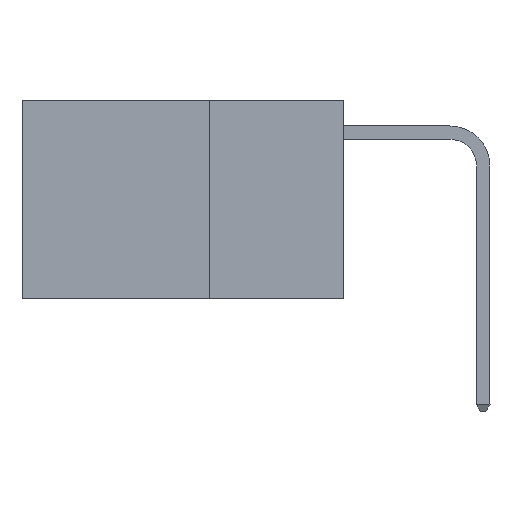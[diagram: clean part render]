
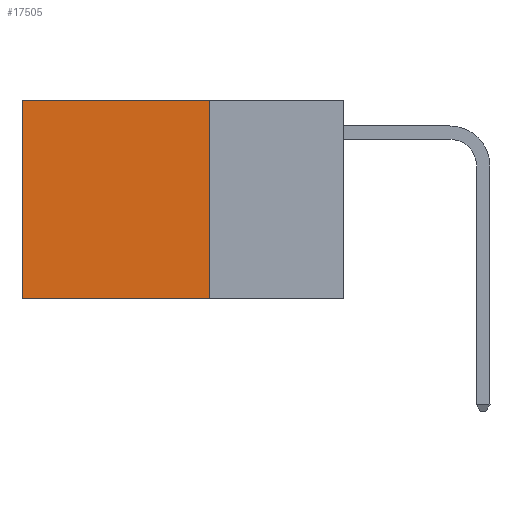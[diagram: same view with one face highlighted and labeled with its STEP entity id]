
A CAD part, left-side view. The second image highlights one B-rep face of the part: STEP entity #17505.
In plain terms, the highlighted planar face has unit normal (-1, 0, 0).
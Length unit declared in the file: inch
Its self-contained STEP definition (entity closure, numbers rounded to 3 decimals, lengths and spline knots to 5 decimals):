
#750 = ORIENTED_EDGE ( 'NONE', *, *, #7232, .T. ) ;
#976 = DIRECTION ( 'NONE',  ( 0., 1., 0. ) ) ;
#1484 = CARTESIAN_POINT ( 'NONE',  ( 0.2625, 0.25, 0. ) ) ;
#1677 = EDGE_LOOP ( 'NONE', ( #3420, #1720, #18262, #750 ) ) ;
#1720 = ORIENTED_EDGE ( 'NONE', *, *, #10864, .F. ) ;
#2090 = DIRECTION ( 'NONE',  ( 0., 0., -1. ) ) ;
#2219 = VECTOR ( 'NONE', #6518, 39.37008 ) ;
#2546 = DIRECTION ( 'NONE',  ( 0., 0., -1. ) ) ;
#3048 = EDGE_CURVE ( 'NONE', #16679, #12373, #3221, .T. ) ;
#3221 = LINE ( 'NONE', #1484, #13771 ) ;
#3420 = ORIENTED_EDGE ( 'NONE', *, *, #5578, .T. ) ;
#4924 = CARTESIAN_POINT ( 'NONE',  ( 0.2625, 0.25, -0.37 ) ) ;
#5212 = VECTOR ( 'NONE', #976, 39.37008 ) ;
#5578 = EDGE_CURVE ( 'NONE', #10657, #12226, #16184, .T. ) ;
#6518 = DIRECTION ( 'NONE',  ( 0., 1., 0. ) ) ;
#6612 = CARTESIAN_POINT ( 'NONE',  ( 0.2625, 0.25, 0. ) ) ;
#7232 = EDGE_CURVE ( 'NONE', #16679, #10657, #10611, .T. ) ;
#9520 = DIRECTION ( 'NONE',  ( 1., 0., 0. ) ) ;
#10611 = LINE ( 'NONE', #6612, #2219 ) ;
#10657 = VERTEX_POINT ( 'NONE', #17568 ) ;
#10864 = EDGE_CURVE ( 'NONE', #12373, #12226, #16834, .T. ) ;
#12226 = VERTEX_POINT ( 'NONE', #16490 ) ;
#12373 = VERTEX_POINT ( 'NONE', #4924 ) ;
#13676 = CARTESIAN_POINT ( 'NONE',  ( 0.2625, 0.25, -0.37 ) ) ;
#13681 = FACE_OUTER_BOUND ( 'NONE', #1677, .T. ) ;
#13771 = VECTOR ( 'NONE', #17239, 39.37008 ) ;
#14792 = CARTESIAN_POINT ( 'NONE',  ( 0.2625, 0.6, 0. ) ) ;
#15456 = CARTESIAN_POINT ( 'NONE',  ( 0.2625, 0.25, 0. ) ) ;
#15756 = VECTOR ( 'NONE', #2090, 39.37008 ) ;
#16032 = AXIS2_PLACEMENT_3D ( 'NONE', #15456, #9520, #2546 ) ;
#16184 = LINE ( 'NONE', #14792, #15756 ) ;
#16490 = CARTESIAN_POINT ( 'NONE',  ( 0.2625, 0.6, -0.37 ) ) ;
#16679 = VERTEX_POINT ( 'NONE', #17502 ) ;
#16751 = PLANE ( 'NONE',  #16032 ) ;
#16834 = LINE ( 'NONE', #13676, #5212 ) ;
#17239 = DIRECTION ( 'NONE',  ( 0., 0., -1. ) ) ;
#17502 = CARTESIAN_POINT ( 'NONE',  ( 0.2625, 0.25, 0. ) ) ;
#17505 = ADVANCED_FACE ( 'NONE', ( #13681 ), #16751, .F. ) ;
#17568 = CARTESIAN_POINT ( 'NONE',  ( 0.2625, 0.6, 0. ) ) ;
#18262 = ORIENTED_EDGE ( 'NONE', *, *, #3048, .F. ) ;
